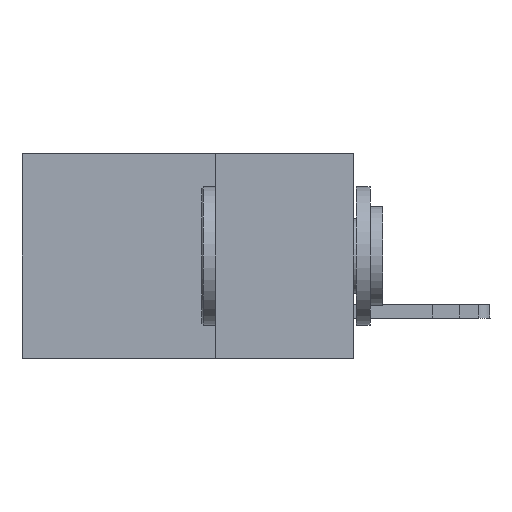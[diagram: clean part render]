
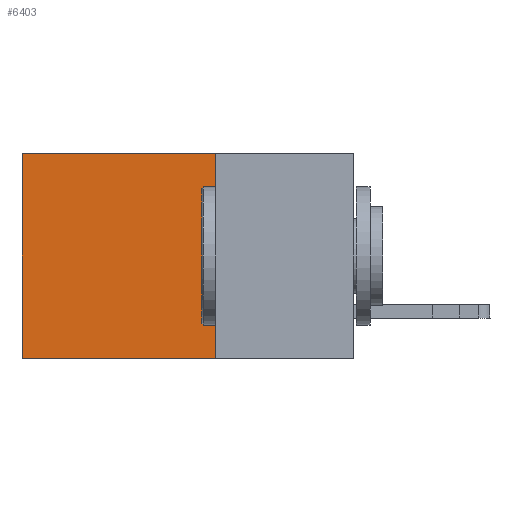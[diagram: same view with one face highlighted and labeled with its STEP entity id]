
A CAD part, left-side view. The second image highlights one B-rep face of the part: STEP entity #6403.
In plain terms, the highlighted planar face has unit normal (-1, 0, 0).
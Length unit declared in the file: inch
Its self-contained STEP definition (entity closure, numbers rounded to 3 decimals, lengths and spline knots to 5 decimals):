
#649 = CARTESIAN_POINT ( 'NONE',  ( 0.2875, 0.25, -0.37 ) ) ;
#860 = PLANE ( 'NONE',  #14235 ) ;
#1314 = DIRECTION ( 'NONE',  ( 0., 0., -1. ) ) ;
#3531 = ORIENTED_EDGE ( 'NONE', *, *, #12467, .F. ) ;
#4002 = VECTOR ( 'NONE', #24197, 39.37008 ) ;
#6403 = ADVANCED_FACE ( 'NONE', ( #8041 ), #860, .F. ) ;
#6417 = EDGE_CURVE ( 'NONE', #27089, #23701, #20869, .T. ) ;
#8041 = FACE_OUTER_BOUND ( 'NONE', #29497, .T. ) ;
#8131 = CARTESIAN_POINT ( 'NONE',  ( 0.2875, 0.6, 0. ) ) ;
#11153 = LINE ( 'NONE', #29558, #29437 ) ;
#12467 = EDGE_CURVE ( 'NONE', #29479, #27089, #11153, .T. ) ;
#13242 = VERTEX_POINT ( 'NONE', #8131 ) ;
#13345 = CARTESIAN_POINT ( 'NONE',  ( 0.2875, 0.25, 0. ) ) ;
#14235 = AXIS2_PLACEMENT_3D ( 'NONE', #26269, #24093, #26677 ) ;
#14421 = LINE ( 'NONE', #29567, #22139 ) ;
#15891 = CARTESIAN_POINT ( 'NONE',  ( 0.2875, 0.6, -0.37 ) ) ;
#16630 = LINE ( 'NONE', #17579, #18855 ) ;
#17579 = CARTESIAN_POINT ( 'NONE',  ( 0.2875, 0.25, 0. ) ) ;
#17631 = ORIENTED_EDGE ( 'NONE', *, *, #18023, .T. ) ;
#18023 = EDGE_CURVE ( 'NONE', #29479, #13242, #16630, .T. ) ;
#18083 = EDGE_CURVE ( 'NONE', #13242, #23701, #14421, .T. ) ;
#18855 = VECTOR ( 'NONE', #24543, 39.37008 ) ;
#20869 = LINE ( 'NONE', #649, #4002 ) ;
#22105 = ORIENTED_EDGE ( 'NONE', *, *, #6417, .F. ) ;
#22139 = VECTOR ( 'NONE', #1314, 39.37008 ) ;
#22405 = DIRECTION ( 'NONE',  ( 0., 0., -1. ) ) ;
#23701 = VERTEX_POINT ( 'NONE', #15891 ) ;
#24093 = DIRECTION ( 'NONE',  ( 1., 0., 0. ) ) ;
#24197 = DIRECTION ( 'NONE',  ( 0., 1., 0. ) ) ;
#24543 = DIRECTION ( 'NONE',  ( 0., 1., 0. ) ) ;
#26269 = CARTESIAN_POINT ( 'NONE',  ( 0.2875, 0.25, 0. ) ) ;
#26677 = DIRECTION ( 'NONE',  ( 0., 0., -1. ) ) ;
#27089 = VERTEX_POINT ( 'NONE', #29027 ) ;
#28824 = ORIENTED_EDGE ( 'NONE', *, *, #18083, .T. ) ;
#29027 = CARTESIAN_POINT ( 'NONE',  ( 0.2875, 0.25, -0.37 ) ) ;
#29437 = VECTOR ( 'NONE', #22405, 39.37008 ) ;
#29479 = VERTEX_POINT ( 'NONE', #13345 ) ;
#29497 = EDGE_LOOP ( 'NONE', ( #28824, #22105, #3531, #17631 ) ) ;
#29558 = CARTESIAN_POINT ( 'NONE',  ( 0.2875, 0.25, 0. ) ) ;
#29567 = CARTESIAN_POINT ( 'NONE',  ( 0.2875, 0.6, 0. ) ) ;
